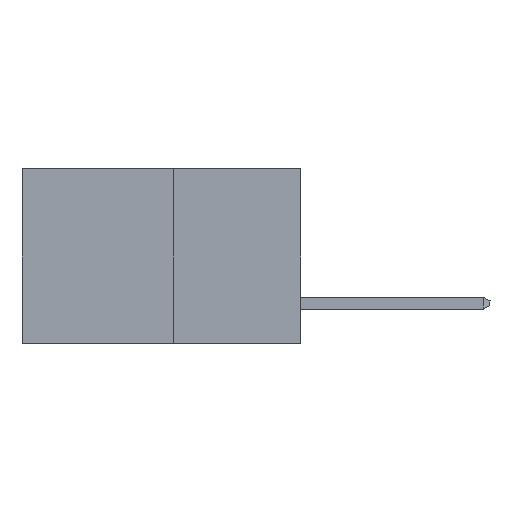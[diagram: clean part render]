
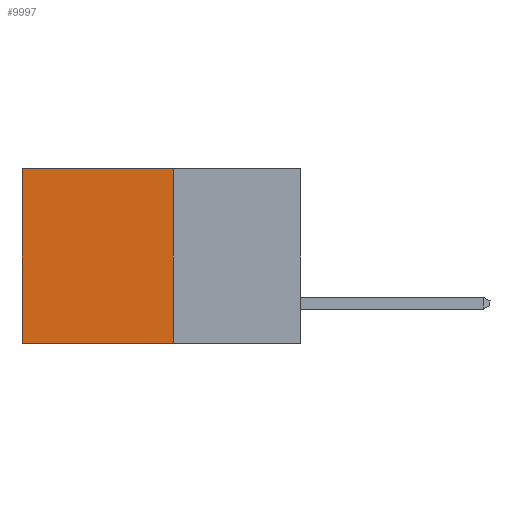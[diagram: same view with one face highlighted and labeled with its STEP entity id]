
A CAD part, left-side view. The second image highlights one B-rep face of the part: STEP entity #9997.
In plain terms, the highlighted planar face has unit normal (-1, 0, 0).
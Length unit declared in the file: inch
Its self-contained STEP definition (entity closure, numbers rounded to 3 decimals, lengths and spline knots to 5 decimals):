
#642 = DIRECTION ( 'NONE',  ( 0., 1., 0. ) ) ;
#715 = CARTESIAN_POINT ( 'NONE',  ( 0.277, 0.59, -0.37 ) ) ;
#864 = LINE ( 'NONE', #9001, #1544 ) ;
#1544 = VECTOR ( 'NONE', #22140, 39.37008 ) ;
#1603 = VECTOR ( 'NONE', #642, 39.37008 ) ;
#2000 = CARTESIAN_POINT ( 'NONE',  ( 0.277, 0.27, 0. ) ) ;
#2277 = LINE ( 'NONE', #11607, #1603 ) ;
#2552 = VECTOR ( 'NONE', #8487, 39.37008 ) ;
#2764 = VECTOR ( 'NONE', #26220, 39.37008 ) ;
#3253 = CARTESIAN_POINT ( 'NONE',  ( 0.277, 0.27, -0.37 ) ) ;
#3277 = LINE ( 'NONE', #17172, #2552 ) ;
#3320 = CARTESIAN_POINT ( 'NONE',  ( 0.277, 0.59, 0. ) ) ;
#6447 = CARTESIAN_POINT ( 'NONE',  ( 0.277, 0.27, -0.37 ) ) ;
#6486 = FACE_OUTER_BOUND ( 'NONE', #18264, .T. ) ;
#6498 = VERTEX_POINT ( 'NONE', #715 ) ;
#8487 = DIRECTION ( 'NONE',  ( 0., 0., -1. ) ) ;
#8645 = ORIENTED_EDGE ( 'NONE', *, *, #21771, .F. ) ;
#8663 = VERTEX_POINT ( 'NONE', #2000 ) ;
#8875 = VERTEX_POINT ( 'NONE', #3320 ) ;
#9001 = CARTESIAN_POINT ( 'NONE',  ( 0.277, 0.27, 0. ) ) ;
#9997 = ADVANCED_FACE ( 'NONE', ( #6486 ), #19553, .F. ) ;
#10403 = AXIS2_PLACEMENT_3D ( 'NONE', #26216, #13071, #28444 ) ;
#11607 = CARTESIAN_POINT ( 'NONE',  ( 0.277, 0.27, -0.37 ) ) ;
#12510 = EDGE_CURVE ( 'NONE', #8663, #8875, #864, .T. ) ;
#13071 = DIRECTION ( 'NONE',  ( 1., 0., 0. ) ) ;
#15637 = ORIENTED_EDGE ( 'NONE', *, *, #26383, .T. ) ;
#17172 = CARTESIAN_POINT ( 'NONE',  ( 0.277, 0.59, -0.37 ) ) ;
#18264 = EDGE_LOOP ( 'NONE', ( #15637, #22623, #8645, #25952 ) ) ;
#19553 = PLANE ( 'NONE',  #10403 ) ;
#21771 = EDGE_CURVE ( 'NONE', #8663, #28186, #26150, .T. ) ;
#22140 = DIRECTION ( 'NONE',  ( 0., 1., 0. ) ) ;
#22623 = ORIENTED_EDGE ( 'NONE', *, *, #25377, .F. ) ;
#25377 = EDGE_CURVE ( 'NONE', #28186, #6498, #2277, .T. ) ;
#25952 = ORIENTED_EDGE ( 'NONE', *, *, #12510, .T. ) ;
#26150 = LINE ( 'NONE', #6447, #2764 ) ;
#26216 = CARTESIAN_POINT ( 'NONE',  ( 0.277, 0.27, -0.37 ) ) ;
#26220 = DIRECTION ( 'NONE',  ( 0., 0., -1. ) ) ;
#26383 = EDGE_CURVE ( 'NONE', #8875, #6498, #3277, .T. ) ;
#28186 = VERTEX_POINT ( 'NONE', #3253 ) ;
#28444 = DIRECTION ( 'NONE',  ( 0., 0., -1. ) ) ;
